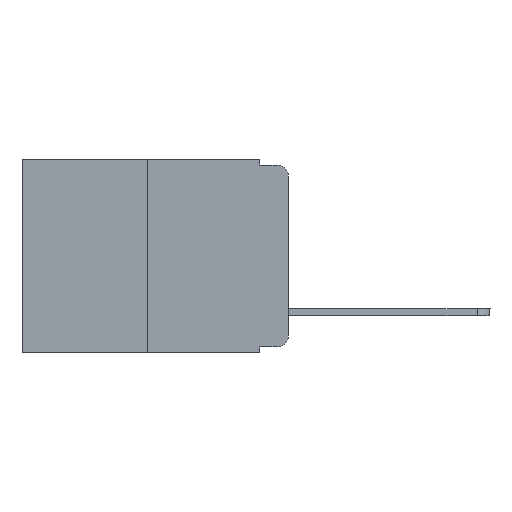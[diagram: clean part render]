
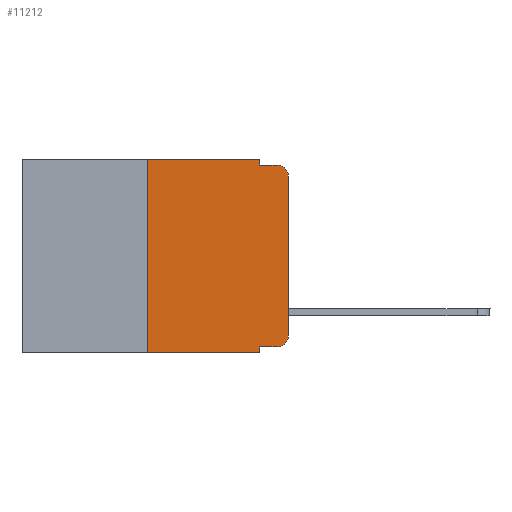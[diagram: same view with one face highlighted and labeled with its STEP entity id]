
A CAD part, left-side view. The second image highlights one B-rep face of the part: STEP entity #11212.
In plain terms, the highlighted planar face has unit normal (-1, 0, 0).
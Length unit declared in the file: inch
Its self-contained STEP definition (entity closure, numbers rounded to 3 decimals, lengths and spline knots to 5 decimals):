
#19 = ORIENTED_EDGE ( 'NONE', *, *, #8150, .T. ) ;
#53 = CARTESIAN_POINT ( 'NONE',  ( 0., 0., -0.313 ) ) ;
#353 = EDGE_CURVE ( 'NONE', #16011, #3694, #9750, .T. ) ;
#439 = CARTESIAN_POINT ( 'NONE',  ( 0., 0.473, -0.343 ) ) ;
#847 = ORIENTED_EDGE ( 'NONE', *, *, #7258, .F. ) ;
#973 = VECTOR ( 'NONE', #20138, 39.37008 ) ;
#1024 = AXIS2_PLACEMENT_3D ( 'NONE', #6022, #16771, #8976 ) ;
#1303 = FACE_OUTER_BOUND ( 'NONE', #18608, .T. ) ;
#1440 = VECTOR ( 'NONE', #10761, 39.37008 ) ;
#2464 = DIRECTION ( 'NONE',  ( 0., 0., -1. ) ) ;
#2523 = CARTESIAN_POINT ( 'NONE',  ( 0., 0.25, 0. ) ) ;
#2955 = ORIENTED_EDGE ( 'NONE', *, *, #11950, .T. ) ;
#3246 = LINE ( 'NONE', #10579, #4197 ) ;
#3352 = VERTEX_POINT ( 'NONE', #6759 ) ;
#3694 = VERTEX_POINT ( 'NONE', #13989 ) ;
#3696 = CARTESIAN_POINT ( 'NONE',  ( 0., 0.051, -0.01 ) ) ;
#3923 = DIRECTION ( 'NONE',  ( 0., -1., 0. ) ) ;
#4007 = ORIENTED_EDGE ( 'NONE', *, *, #11259, .F. ) ;
#4197 = VECTOR ( 'NONE', #18562, 39.37008 ) ;
#4783 = EDGE_CURVE ( 'NONE', #3694, #5203, #9530, .T. ) ;
#5203 = VERTEX_POINT ( 'NONE', #11719 ) ;
#5763 = LINE ( 'NONE', #11685, #14843 ) ;
#6022 = CARTESIAN_POINT ( 'NONE',  ( 0., 0.02, -0.313 ) ) ;
#6121 = CARTESIAN_POINT ( 'NONE',  ( 0., 0.051, -0.333 ) ) ;
#6153 = DIRECTION ( 'NONE',  ( -1., 0., 0. ) ) ;
#6289 = VECTOR ( 'NONE', #3923, 39.37008 ) ;
#6466 = ORIENTED_EDGE ( 'NONE', *, *, #13597, .F. ) ;
#6759 = CARTESIAN_POINT ( 'NONE',  ( 0., 0.02, -0.333 ) ) ;
#7258 = EDGE_CURVE ( 'NONE', #11653, #5203, #3246, .T. ) ;
#7586 = DIRECTION ( 'NONE',  ( 0., -1., 0. ) ) ;
#7680 = ORIENTED_EDGE ( 'NONE', *, *, #4783, .T. ) ;
#7977 = EDGE_CURVE ( 'NONE', #19610, #10479, #8036, .T. ) ;
#8036 = LINE ( 'NONE', #18711, #973 ) ;
#8150 = EDGE_CURVE ( 'NONE', #19610, #16309, #9968, .T. ) ;
#8323 = DIRECTION ( 'NONE',  ( 0., 0., -1. ) ) ;
#8389 = EDGE_CURVE ( 'NONE', #11796, #3352, #14369, .T. ) ;
#8881 = CARTESIAN_POINT ( 'NONE',  ( 0., 0.473, 0. ) ) ;
#8885 = EDGE_CURVE ( 'NONE', #11796, #16309, #5763, .T. ) ;
#8976 = DIRECTION ( 'NONE',  ( 0., 0., -1. ) ) ;
#9003 = CARTESIAN_POINT ( 'NONE',  ( 0., 0.473, 0. ) ) ;
#9530 = CIRCLE ( 'NONE', #18777, 0.02 ) ;
#9750 = LINE ( 'NONE', #17536, #10923 ) ;
#9850 = VECTOR ( 'NONE', #8323, 39.37008 ) ;
#9968 = LINE ( 'NONE', #439, #6289 ) ;
#10198 = CARTESIAN_POINT ( 'NONE',  ( 0., 0.051, -0.333 ) ) ;
#10359 = DIRECTION ( 'NONE',  ( 0., 0., -1. ) ) ;
#10479 = VERTEX_POINT ( 'NONE', #2523 ) ;
#10579 = CARTESIAN_POINT ( 'NONE',  ( 0., 0.051, -0.01 ) ) ;
#10761 = DIRECTION ( 'NONE',  ( 0., -1., 0. ) ) ;
#10923 = VECTOR ( 'NONE', #12658, 39.37008 ) ;
#11212 = ADVANCED_FACE ( 'NONE', ( #1303 ), #12109, .F. ) ;
#11259 = EDGE_CURVE ( 'NONE', #10479, #19915, #17414, .T. ) ;
#11410 = ORIENTED_EDGE ( 'NONE', *, *, #8885, .F. ) ;
#11653 = VERTEX_POINT ( 'NONE', #3696 ) ;
#11685 = CARTESIAN_POINT ( 'NONE',  ( 0., 0.051, 0. ) ) ;
#11719 = CARTESIAN_POINT ( 'NONE',  ( 0., 0.02, -0.01 ) ) ;
#11796 = VERTEX_POINT ( 'NONE', #10198 ) ;
#11950 = EDGE_CURVE ( 'NONE', #3352, #16011, #16893, .T. ) ;
#12069 = CARTESIAN_POINT ( 'NONE',  ( 0., 0.25, -0.343 ) ) ;
#12109 = PLANE ( 'NONE',  #15904 ) ;
#12494 = CARTESIAN_POINT ( 'NONE',  ( 0., 0.02, -0.03 ) ) ;
#12658 = DIRECTION ( 'NONE',  ( 0., 0., 1. ) ) ;
#12855 = ORIENTED_EDGE ( 'NONE', *, *, #353, .T. ) ;
#13194 = ORIENTED_EDGE ( 'NONE', *, *, #8389, .T. ) ;
#13388 = CARTESIAN_POINT ( 'NONE',  ( 0., 0.051, 0. ) ) ;
#13597 = EDGE_CURVE ( 'NONE', #19915, #11653, #14279, .T. ) ;
#13989 = CARTESIAN_POINT ( 'NONE',  ( 0., 0., -0.03 ) ) ;
#14279 = LINE ( 'NONE', #14539, #9850 ) ;
#14369 = LINE ( 'NONE', #6121, #1440 ) ;
#14539 = CARTESIAN_POINT ( 'NONE',  ( 0., 0.051, 0. ) ) ;
#14843 = VECTOR ( 'NONE', #2464, 39.37008 ) ;
#15232 = DIRECTION ( 'NONE',  ( 1., 0., 0. ) ) ;
#15454 = VECTOR ( 'NONE', #7586, 39.37008 ) ;
#15854 = ORIENTED_EDGE ( 'NONE', *, *, #7977, .F. ) ;
#15904 = AXIS2_PLACEMENT_3D ( 'NONE', #8881, #15232, #10359 ) ;
#16011 = VERTEX_POINT ( 'NONE', #53 ) ;
#16309 = VERTEX_POINT ( 'NONE', #17836 ) ;
#16771 = DIRECTION ( 'NONE',  ( -1., 0., 0. ) ) ;
#16893 = CIRCLE ( 'NONE', #1024, 0.02 ) ;
#17414 = LINE ( 'NONE', #9003, #15454 ) ;
#17536 = CARTESIAN_POINT ( 'NONE',  ( 0., 0., 0. ) ) ;
#17836 = CARTESIAN_POINT ( 'NONE',  ( 0., 0.051, -0.343 ) ) ;
#18562 = DIRECTION ( 'NONE',  ( 0., -1., 0. ) ) ;
#18608 = EDGE_LOOP ( 'NONE', ( #12855, #7680, #847, #6466, #4007, #15854, #19, #11410, #13194, #2955 ) ) ;
#18653 = DIRECTION ( 'NONE',  ( 0., 0., -1. ) ) ;
#18711 = CARTESIAN_POINT ( 'NONE',  ( 0., 0.25, 0. ) ) ;
#18777 = AXIS2_PLACEMENT_3D ( 'NONE', #12494, #6153, #18653 ) ;
#19610 = VERTEX_POINT ( 'NONE', #12069 ) ;
#19915 = VERTEX_POINT ( 'NONE', #13388 ) ;
#20138 = DIRECTION ( 'NONE',  ( 0., 0., 1. ) ) ;
